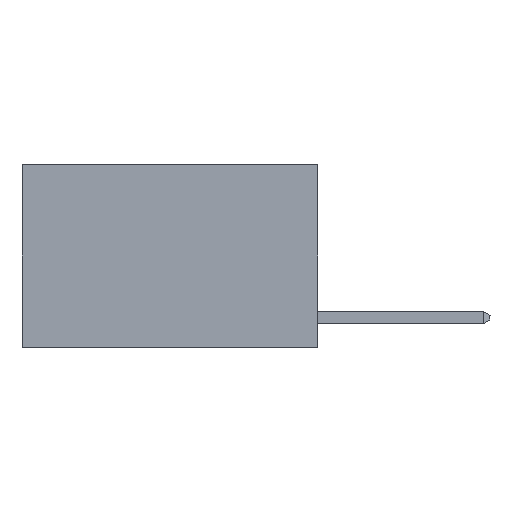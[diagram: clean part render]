
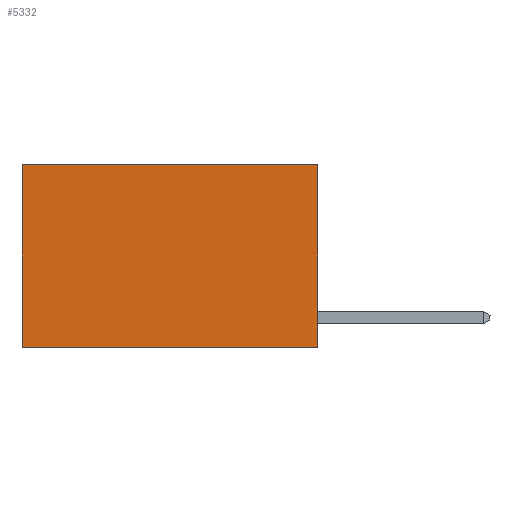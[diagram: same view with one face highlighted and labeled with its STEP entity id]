
A CAD part, left-side view. The second image highlights one B-rep face of the part: STEP entity #5332.
In plain terms, the highlighted planar face has unit normal (-1, 0, 0).
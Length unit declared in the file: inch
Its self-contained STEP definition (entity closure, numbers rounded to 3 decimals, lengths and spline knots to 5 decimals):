
#1694 = VECTOR ( 'NONE', #27705, 39.37008 ) ;
#1935 = CARTESIAN_POINT ( 'NONE',  ( 0.2625, 0., 0. ) ) ;
#1977 = DIRECTION ( 'NONE',  ( 1., 0., 0. ) ) ;
#3076 = LINE ( 'NONE', #18012, #25510 ) ;
#3264 = ORIENTED_EDGE ( 'NONE', *, *, #22165, .T. ) ;
#4112 = VERTEX_POINT ( 'NONE', #1935 ) ;
#5332 = ADVANCED_FACE ( 'NONE', ( #16248 ), #12765, .F. ) ;
#7537 = LINE ( 'NONE', #21210, #1694 ) ;
#9644 = EDGE_CURVE ( 'NONE', #22685, #28220, #7537, .T. ) ;
#9738 = VECTOR ( 'NONE', #10120, 39.37008 ) ;
#10120 = DIRECTION ( 'NONE',  ( 0., 1., 0. ) ) ;
#11250 = EDGE_LOOP ( 'NONE', ( #12705, #19913, #25693, #3264 ) ) ;
#12705 = ORIENTED_EDGE ( 'NONE', *, *, #9644, .T. ) ;
#12765 = PLANE ( 'NONE',  #13464 ) ;
#13464 = AXIS2_PLACEMENT_3D ( 'NONE', #27967, #1977, #17177 ) ;
#14550 = DIRECTION ( 'NONE',  ( 0., 1., 0. ) ) ;
#16102 = CARTESIAN_POINT ( 'NONE',  ( 0.2625, 0.6, 0. ) ) ;
#16248 = FACE_OUTER_BOUND ( 'NONE', #11250, .T. ) ;
#17177 = DIRECTION ( 'NONE',  ( 0., 0., -1. ) ) ;
#17991 = CARTESIAN_POINT ( 'NONE',  ( 0.2625, 0.6, -0.37 ) ) ;
#18012 = CARTESIAN_POINT ( 'NONE',  ( 0.2625, 0., 0. ) ) ;
#18188 = LINE ( 'NONE', #21141, #23974 ) ;
#18799 = CARTESIAN_POINT ( 'NONE',  ( 0.2625, 0., 0. ) ) ;
#19913 = ORIENTED_EDGE ( 'NONE', *, *, #22923, .F. ) ;
#20175 = EDGE_CURVE ( 'NONE', #4112, #21675, #3076, .T. ) ;
#21141 = CARTESIAN_POINT ( 'NONE',  ( 0.2625, 0., -0.37 ) ) ;
#21210 = CARTESIAN_POINT ( 'NONE',  ( 0.2625, 0.6, 0. ) ) ;
#21672 = CARTESIAN_POINT ( 'NONE',  ( 0.2625, 0., -0.37 ) ) ;
#21675 = VERTEX_POINT ( 'NONE', #21672 ) ;
#22165 = EDGE_CURVE ( 'NONE', #4112, #22685, #26379, .T. ) ;
#22685 = VERTEX_POINT ( 'NONE', #16102 ) ;
#22923 = EDGE_CURVE ( 'NONE', #21675, #28220, #18188, .T. ) ;
#23974 = VECTOR ( 'NONE', #14550, 39.37008 ) ;
#25510 = VECTOR ( 'NONE', #26727, 39.37008 ) ;
#25693 = ORIENTED_EDGE ( 'NONE', *, *, #20175, .F. ) ;
#26379 = LINE ( 'NONE', #18799, #9738 ) ;
#26727 = DIRECTION ( 'NONE',  ( 0., 0., -1. ) ) ;
#27705 = DIRECTION ( 'NONE',  ( 0., 0., -1. ) ) ;
#27967 = CARTESIAN_POINT ( 'NONE',  ( 0.2625, 0., 0. ) ) ;
#28220 = VERTEX_POINT ( 'NONE', #17991 ) ;
